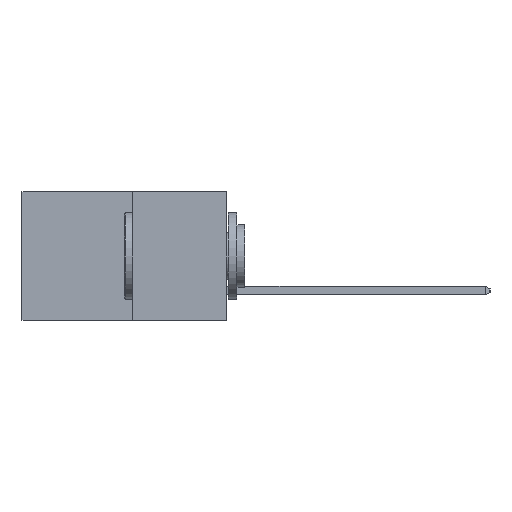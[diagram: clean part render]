
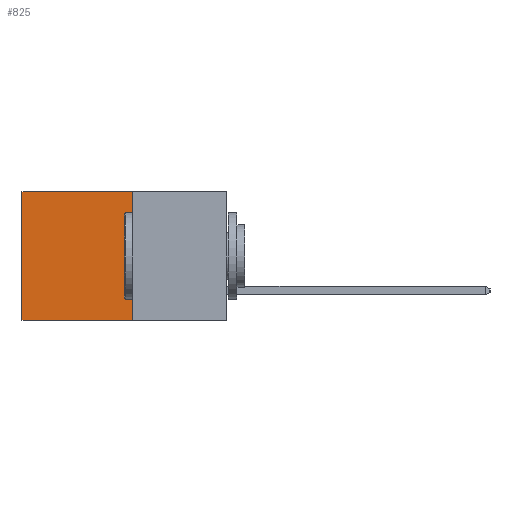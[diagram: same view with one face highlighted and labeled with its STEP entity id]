
A CAD part, left-side view. The second image highlights one B-rep face of the part: STEP entity #825.
In plain terms, the highlighted planar face has unit normal (-1, 0, 0).
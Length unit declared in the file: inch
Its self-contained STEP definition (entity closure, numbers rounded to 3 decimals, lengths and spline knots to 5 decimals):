
#825 = ADVANCED_FACE ( 'NONE', ( #1935 ), #6306, .F. ) ;
#1724 = LINE ( 'NONE', #7715, #6081 ) ;
#1935 = FACE_OUTER_BOUND ( 'NONE', #4968, .T. ) ;
#1954 = DIRECTION ( 'NONE',  ( 0., 0., -1. ) ) ;
#2298 = DIRECTION ( 'NONE',  ( 0., 1., 0. ) ) ;
#2736 = VECTOR ( 'NONE', #2298, 39.37008 ) ;
#2987 = LINE ( 'NONE', #3700, #2736 ) ;
#3005 = ORIENTED_EDGE ( 'NONE', *, *, #5537, .T. ) ;
#3290 = CARTESIAN_POINT ( 'NONE',  ( 0.277, 0.27, 0. ) ) ;
#3370 = VERTEX_POINT ( 'NONE', #8660 ) ;
#3393 = CARTESIAN_POINT ( 'NONE',  ( 0.277, 0.59, -0.37 ) ) ;
#3700 = CARTESIAN_POINT ( 'NONE',  ( 0.277, 0.27, 0. ) ) ;
#3814 = DIRECTION ( 'NONE',  ( 0., 1., 0. ) ) ;
#4954 = LINE ( 'NONE', #9737, #8813 ) ;
#4968 = EDGE_LOOP ( 'NONE', ( #3005, #7202, #9236, #5406 ) ) ;
#5243 = VECTOR ( 'NONE', #5511, 39.37008 ) ;
#5406 = ORIENTED_EDGE ( 'NONE', *, *, #9816, .T. ) ;
#5448 = EDGE_CURVE ( 'NONE', #8017, #7525, #1724, .T. ) ;
#5511 = DIRECTION ( 'NONE',  ( 0., 0., -1. ) ) ;
#5537 = EDGE_CURVE ( 'NONE', #3370, #7525, #5741, .T. ) ;
#5741 = LINE ( 'NONE', #10070, #5243 ) ;
#5974 = AXIS2_PLACEMENT_3D ( 'NONE', #7873, #9504, #9834 ) ;
#6081 = VECTOR ( 'NONE', #3814, 39.37008 ) ;
#6306 = PLANE ( 'NONE',  #5974 ) ;
#7202 = ORIENTED_EDGE ( 'NONE', *, *, #5448, .F. ) ;
#7457 = VERTEX_POINT ( 'NONE', #3290 ) ;
#7525 = VERTEX_POINT ( 'NONE', #3393 ) ;
#7653 = EDGE_CURVE ( 'NONE', #7457, #8017, #4954, .T. ) ;
#7715 = CARTESIAN_POINT ( 'NONE',  ( 0.277, 0.27, -0.37 ) ) ;
#7873 = CARTESIAN_POINT ( 'NONE',  ( 0.277, 0.27, -0.37 ) ) ;
#8017 = VERTEX_POINT ( 'NONE', #9266 ) ;
#8660 = CARTESIAN_POINT ( 'NONE',  ( 0.277, 0.59, 0. ) ) ;
#8813 = VECTOR ( 'NONE', #1954, 39.37008 ) ;
#9236 = ORIENTED_EDGE ( 'NONE', *, *, #7653, .F. ) ;
#9266 = CARTESIAN_POINT ( 'NONE',  ( 0.277, 0.27, -0.37 ) ) ;
#9504 = DIRECTION ( 'NONE',  ( 1., 0., 0. ) ) ;
#9737 = CARTESIAN_POINT ( 'NONE',  ( 0.277, 0.27, -0.37 ) ) ;
#9816 = EDGE_CURVE ( 'NONE', #7457, #3370, #2987, .T. ) ;
#9834 = DIRECTION ( 'NONE',  ( 0., 0., -1. ) ) ;
#10070 = CARTESIAN_POINT ( 'NONE',  ( 0.277, 0.59, -0.37 ) ) ;
